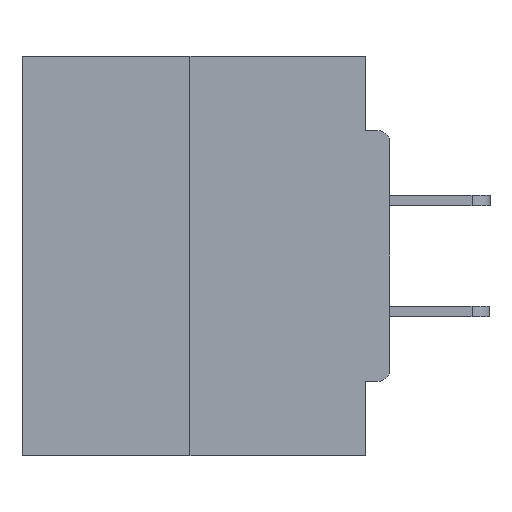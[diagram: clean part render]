
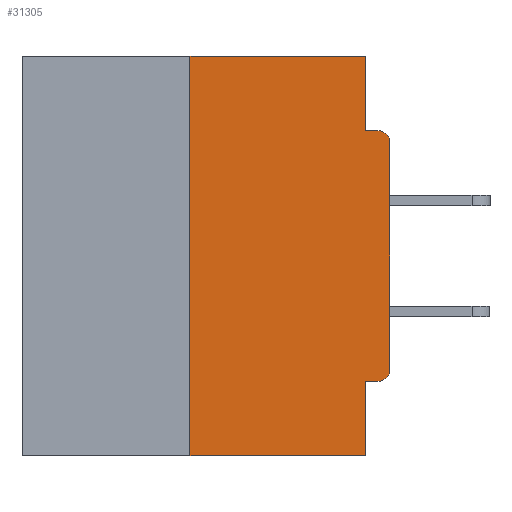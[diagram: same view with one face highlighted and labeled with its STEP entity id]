
A CAD part, left-side view. The second image highlights one B-rep face of the part: STEP entity #31305.
In plain terms, the highlighted planar face has unit normal (-1, 0, 0).
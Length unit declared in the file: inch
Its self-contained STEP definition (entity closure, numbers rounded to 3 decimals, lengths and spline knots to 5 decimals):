
#187 = LINE ( 'NONE', #32856, #28552 ) ;
#1711 = VECTOR ( 'NONE', #13656, 39.37008 ) ;
#1741 = VERTEX_POINT ( 'NONE', #13172 ) ;
#2381 = DIRECTION ( 'NONE',  ( -1., 0., 0. ) ) ;
#2405 = ORIENTED_EDGE ( 'NONE', *, *, #14304, .F. ) ;
#2699 = VERTEX_POINT ( 'NONE', #9466 ) ;
#2721 = DIRECTION ( 'NONE',  ( 0., 0., -1. ) ) ;
#3058 = DIRECTION ( 'NONE',  ( 0., 0., -1. ) ) ;
#3434 = CARTESIAN_POINT ( 'NONE',  ( 0., 0., -0.3915 ) ) ;
#3708 = ORIENTED_EDGE ( 'NONE', *, *, #7895, .T. ) ;
#4041 = LINE ( 'NONE', #26230, #24170 ) ;
#4269 = ORIENTED_EDGE ( 'NONE', *, *, #15052, .F. ) ;
#4763 = LINE ( 'NONE', #8005, #33524 ) ;
#5548 = VECTOR ( 'NONE', #20814, 39.37008 ) ;
#5637 = CARTESIAN_POINT ( 'NONE',  ( 0., 0.031, -0.0935 ) ) ;
#6352 = DIRECTION ( 'NONE',  ( 0., 0., 1. ) ) ;
#6768 = DIRECTION ( 'NONE',  ( 0., 0., -1. ) ) ;
#6998 = PLANE ( 'NONE',  #32338 ) ;
#7168 = DIRECTION ( 'NONE',  ( 0., 0., -1. ) ) ;
#7895 = EDGE_CURVE ( 'NONE', #23382, #2699, #4763, .T. ) ;
#8005 = CARTESIAN_POINT ( 'NONE',  ( 0., 0.46, -0.5 ) ) ;
#9466 = CARTESIAN_POINT ( 'NONE',  ( 0., 0.031, -0.5 ) ) ;
#9891 = CARTESIAN_POINT ( 'NONE',  ( 0., 0.25, -0.5 ) ) ;
#10058 = VERTEX_POINT ( 'NONE', #15009 ) ;
#10236 = EDGE_CURVE ( 'NONE', #23382, #17166, #14818, .T. ) ;
#10364 = DIRECTION ( 'NONE',  ( 0., 0., -1. ) ) ;
#10837 = CARTESIAN_POINT ( 'NONE',  ( 0., 0.015, -0.1085 ) ) ;
#10936 = DIRECTION ( 'NONE',  ( 0., -1., 0. ) ) ;
#11333 = AXIS2_PLACEMENT_3D ( 'NONE', #26255, #21455, #3058 ) ;
#11925 = VERTEX_POINT ( 'NONE', #17452 ) ;
#12243 = CARTESIAN_POINT ( 'NONE',  ( 0., 0.46, 0. ) ) ;
#12413 = CARTESIAN_POINT ( 'NONE',  ( 0., 0.031, 0. ) ) ;
#12503 = LINE ( 'NONE', #18150, #5548 ) ;
#13172 = CARTESIAN_POINT ( 'NONE',  ( 0., 0., -0.1085 ) ) ;
#13656 = DIRECTION ( 'NONE',  ( 0., 0., 1. ) ) ;
#14011 = VERTEX_POINT ( 'NONE', #5637 ) ;
#14304 = EDGE_CURVE ( 'NONE', #10058, #23633, #33265, .T. ) ;
#14818 = LINE ( 'NONE', #21251, #1711 ) ;
#15009 = CARTESIAN_POINT ( 'NONE',  ( 0., 0.015, -0.4065 ) ) ;
#15052 = EDGE_CURVE ( 'NONE', #14011, #11925, #16775, .T. ) ;
#16775 = LINE ( 'NONE', #24445, #19671 ) ;
#17128 = EDGE_CURVE ( 'NONE', #10058, #31039, #30640, .T. ) ;
#17166 = VERTEX_POINT ( 'NONE', #24534 ) ;
#17452 = CARTESIAN_POINT ( 'NONE',  ( 0., 0.015, -0.0935 ) ) ;
#17482 = ORIENTED_EDGE ( 'NONE', *, *, #17128, .T. ) ;
#17514 = CIRCLE ( 'NONE', #21896, 0.015 ) ;
#17900 = CARTESIAN_POINT ( 'NONE',  ( 0., 0.031, 0. ) ) ;
#18150 = CARTESIAN_POINT ( 'NONE',  ( 0., 0.46, 0. ) ) ;
#18267 = EDGE_CURVE ( 'NONE', #23633, #2699, #4041, .T. ) ;
#19671 = VECTOR ( 'NONE', #29602, 39.37008 ) ;
#20028 = EDGE_CURVE ( 'NONE', #17166, #25967, #12503, .T. ) ;
#20814 = DIRECTION ( 'NONE',  ( 0., -1., 0. ) ) ;
#21197 = ORIENTED_EDGE ( 'NONE', *, *, #23938, .F. ) ;
#21251 = CARTESIAN_POINT ( 'NONE',  ( 0., 0.25, 0. ) ) ;
#21455 = DIRECTION ( 'NONE',  ( -1., 0., 0. ) ) ;
#21624 = ORIENTED_EDGE ( 'NONE', *, *, #27451, .T. ) ;
#21896 = AXIS2_PLACEMENT_3D ( 'NONE', #10837, #2381, #2721 ) ;
#22422 = ORIENTED_EDGE ( 'NONE', *, *, #26188, .T. ) ;
#22461 = CARTESIAN_POINT ( 'NONE',  ( 0., 0., -0.4065 ) ) ;
#22617 = LINE ( 'NONE', #12413, #25899 ) ;
#23382 = VERTEX_POINT ( 'NONE', #9891 ) ;
#23595 = ORIENTED_EDGE ( 'NONE', *, *, #20028, .F. ) ;
#23633 = VERTEX_POINT ( 'NONE', #24597 ) ;
#23938 = EDGE_CURVE ( 'NONE', #25967, #14011, #22617, .T. ) ;
#24170 = VECTOR ( 'NONE', #10364, 39.37008 ) ;
#24445 = CARTESIAN_POINT ( 'NONE',  ( 0., 0., -0.0935 ) ) ;
#24534 = CARTESIAN_POINT ( 'NONE',  ( 0., 0.25, 0. ) ) ;
#24597 = CARTESIAN_POINT ( 'NONE',  ( 0., 0.031, -0.4065 ) ) ;
#25090 = DIRECTION ( 'NONE',  ( 0., 1., 0. ) ) ;
#25899 = VECTOR ( 'NONE', #7168, 39.37008 ) ;
#25967 = VERTEX_POINT ( 'NONE', #17900 ) ;
#26188 = EDGE_CURVE ( 'NONE', #1741, #11925, #17514, .T. ) ;
#26213 = ORIENTED_EDGE ( 'NONE', *, *, #10236, .F. ) ;
#26230 = CARTESIAN_POINT ( 'NONE',  ( 0., 0.031, -0.5 ) ) ;
#26255 = CARTESIAN_POINT ( 'NONE',  ( 0., 0.015, -0.3915 ) ) ;
#27451 = EDGE_CURVE ( 'NONE', #31039, #1741, #187, .T. ) ;
#28552 = VECTOR ( 'NONE', #6352, 39.37008 ) ;
#29602 = DIRECTION ( 'NONE',  ( 0., -1., 0. ) ) ;
#30020 = EDGE_LOOP ( 'NONE', ( #23595, #26213, #3708, #30365, #2405, #17482, #21624, #22422, #4269, #21197 ) ) ;
#30365 = ORIENTED_EDGE ( 'NONE', *, *, #18267, .F. ) ;
#30640 = CIRCLE ( 'NONE', #11333, 0.015 ) ;
#31039 = VERTEX_POINT ( 'NONE', #3434 ) ;
#31305 = ADVANCED_FACE ( 'NONE', ( #32688 ), #6998, .F. ) ;
#32338 = AXIS2_PLACEMENT_3D ( 'NONE', #12243, #32934, #6768 ) ;
#32688 = FACE_OUTER_BOUND ( 'NONE', #30020, .T. ) ;
#32856 = CARTESIAN_POINT ( 'NONE',  ( 0., 0., 0. ) ) ;
#32934 = DIRECTION ( 'NONE',  ( 1., 0., 0. ) ) ;
#33265 = LINE ( 'NONE', #22461, #33690 ) ;
#33524 = VECTOR ( 'NONE', #10936, 39.37008 ) ;
#33690 = VECTOR ( 'NONE', #25090, 39.37008 ) ;
